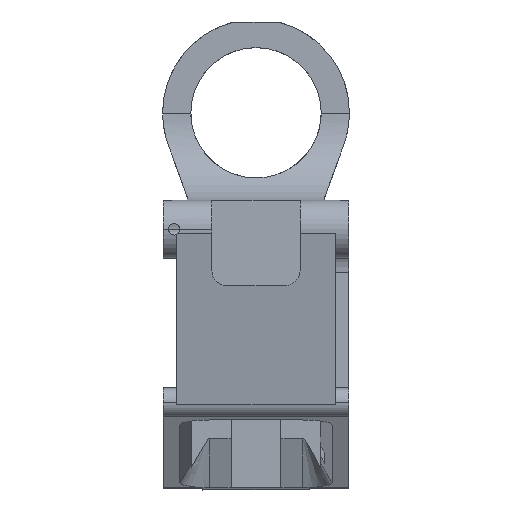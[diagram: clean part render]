
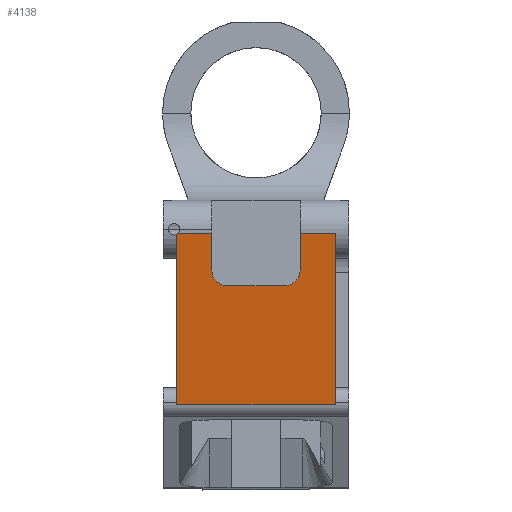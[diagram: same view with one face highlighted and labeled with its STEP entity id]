
A CAD part, top view. The second image highlights one B-rep face of the part: STEP entity #4138.
In plain terms, the highlighted planar face has unit normal (0, -0.156, 0.988).
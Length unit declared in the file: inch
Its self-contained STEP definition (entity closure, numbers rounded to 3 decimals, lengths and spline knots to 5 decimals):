
#20 = CARTESIAN_POINT ( 'NONE',  ( -0.67032, -0.28911, 8.96692 ) ) ;
#81 = EDGE_LOOP ( 'NONE', ( #6582, #3793, #6591, #2601, #5890, #3382, #1505, #7975, #5842, #2264, #7993 ) ) ;
#239 = EDGE_CURVE ( 'NONE', #453, #8430, #6435, .T. ) ;
#329 = DIRECTION ( 'NONE',  ( 0., -0.988, -0.156 ) ) ;
#437 = CARTESIAN_POINT ( 'NONE',  ( 0.675, -1.01855, 8.85139 ) ) ;
#453 = VERTEX_POINT ( 'NONE', #8779 ) ;
#576 = CARTESIAN_POINT ( 'NONE',  ( -0.376, -0.605, 8.91689 ) ) ;
#686 = VERTEX_POINT ( 'NONE', #1953 ) ;
#732 = VERTEX_POINT ( 'NONE', #1987 ) ;
#1032 = EDGE_CURVE ( 'NONE', #8430, #732, #4362, .T. ) ;
#1067 = FACE_OUTER_BOUND ( 'NONE', #81, .T. ) ;
#1092 = CARTESIAN_POINT ( 'NONE',  ( -0.675, -1.74799, 8.73586 ) ) ;
#1142 = CARTESIAN_POINT ( 'NONE',  ( -0.675, -0.29215, 8.96643 ) ) ;
#1505 = ORIENTED_EDGE ( 'NONE', *, *, #6624, .T. ) ;
#1625 = DIRECTION ( 'NONE',  ( 1., 0., 0. ) ) ;
#1953 = CARTESIAN_POINT ( 'NONE',  ( 0.675, -0.28911, 8.96692 ) ) ;
#1987 = CARTESIAN_POINT ( 'NONE',  ( -0.251, -0.73, 8.89709 ) ) ;
#2120 = CARTESIAN_POINT ( 'NONE',  ( 0.376, -0.28911, 8.96692 ) ) ;
#2230 = VERTEX_POINT ( 'NONE', #7194 ) ;
#2264 = ORIENTED_EDGE ( 'NONE', *, *, #239, .T. ) ;
#2399 = VECTOR ( 'NONE', #8054, 39.37008 ) ;
#2515 = CARTESIAN_POINT ( 'NONE',  ( -0.675, -0.28911, 8.96692 ) ) ;
#2586 = CARTESIAN_POINT ( 'NONE',  ( 0.675, -1.74799, 8.73586 ) ) ;
#2601 = ORIENTED_EDGE ( 'NONE', *, *, #8705, .T. ) ;
#2766 = CARTESIAN_POINT ( 'NONE',  ( -0.251, -0.73, 8.89709 ) ) ;
#2842 = LINE ( 'NONE', #3835, #3527 ) ;
#2854 = CARTESIAN_POINT ( 'NONE',  ( -0.675, -1.74799, 8.73586 ) ) ;
#2950 = CARTESIAN_POINT ( 'NONE',  ( -0.675, -0.29215, 8.96643 ) ) ;
#3178 = LINE ( 'NONE', #7490, #8582 ) ;
#3382 = ORIENTED_EDGE ( 'NONE', *, *, #5955, .T. ) ;
#3527 = VECTOR ( 'NONE', #1625, 39.37008 ) ;
#3793 = ORIENTED_EDGE ( 'NONE', *, *, #5943, .T. ) ;
#3835 = CARTESIAN_POINT ( 'NONE',  ( 0., -1.74799, 8.73586 ) ) ;
#3979 = PLANE ( 'NONE',  #4815 ) ;
#4124 = CARTESIAN_POINT ( 'NONE',  ( -0.376, -0.605, 8.91689 ) ) ;
#4138 = ADVANCED_FACE ( 'NONE', ( #1067 ), #3979, .T. ) ;
#4331 = DIRECTION ( 'NONE',  ( 0., 0.988, 0.156 ) ) ;
#4334 = CARTESIAN_POINT ( 'NONE',  ( 0., -0.73, 8.89709 ) ) ;
#4347 = CARTESIAN_POINT ( 'NONE',  ( 0.32422, -0.73, 8.89709 ) ) ;
#4362 = LINE ( 'NONE', #4334, #2399 ) ;
#4546 = CARTESIAN_POINT ( 'NONE',  ( -0.376, -0.28911, 8.96692 ) ) ;
#4596 = VECTOR ( 'NONE', #4825, 39.37008 ) ;
#4651 = VERTEX_POINT ( 'NONE', #1142 ) ;
#4663 = LINE ( 'NONE', #7784, #8807 ) ;
#4726 = DIRECTION ( 'NONE',  ( 0., -0.156, 0.988 ) ) ;
#4778 = VERTEX_POINT ( 'NONE', #2120 ) ;
#4786 =( BOUNDED_CURVE ( )  B_SPLINE_CURVE ( 3, ( #20, #5139, #7344, #2950 ),
 .UNSPECIFIED., .F., .F. ) 
 B_SPLINE_CURVE_WITH_KNOTS ( ( 4, 4 ),
 ( 5.65037, 5.76554 ),
 .UNSPECIFIED. ) 
 CURVE ( )  GEOMETRIC_REPRESENTATION_ITEM ( )  RATIONAL_B_SPLINE_CURVE ( ( 1., 0.999, 0.999, 1. ) ) 
 REPRESENTATION_ITEM ( '' )  );
#4815 = AXIS2_PLACEMENT_3D ( 'NONE', #2515, #4726, #329 ) ;
#4825 = DIRECTION ( 'NONE',  ( 0., 0.988, 0.156 ) ) ;
#4944 = VERTEX_POINT ( 'NONE', #8929 ) ;
#4971 = CARTESIAN_POINT ( 'NONE',  ( -0.376, -0.67822, 8.90529 ) ) ;
#5139 = CARTESIAN_POINT ( 'NONE',  ( -0.67182, -0.29021, 8.96675 ) ) ;
#5152 =( BOUNDED_CURVE ( )  B_SPLINE_CURVE ( 3, ( #2766, #7145, #4971, #576 ),
 .UNSPECIFIED., .F., .F. ) 
 B_SPLINE_CURVE_WITH_KNOTS ( ( 4, 4 ),
 ( 3.14159, 4.71239 ),
 .UNSPECIFIED. ) 
 CURVE ( )  GEOMETRIC_REPRESENTATION_ITEM ( )  RATIONAL_B_SPLINE_CURVE ( ( 1., 0.805, 0.805, 1. ) ) 
 REPRESENTATION_ITEM ( '' )  );
#5331 = CARTESIAN_POINT ( 'NONE',  ( 0.58425, -0.28911, 8.96692 ) ) ;
#5630 = EDGE_CURVE ( 'NONE', #2230, #4944, #3178, .T. ) ;
#5828 = CARTESIAN_POINT ( 'NONE',  ( 0.376, -0.605, 8.91689 ) ) ;
#5842 = ORIENTED_EDGE ( 'NONE', *, *, #7772, .F. ) ;
#5890 = ORIENTED_EDGE ( 'NONE', *, *, #9008, .F. ) ;
#5943 = EDGE_CURVE ( 'NONE', #8506, #2230, #8701, .T. ) ;
#5955 = EDGE_CURVE ( 'NONE', #7697, #8208, #2842, .T. ) ;
#6251 = CARTESIAN_POINT ( 'NONE',  ( 0.251, -0.73, 8.89709 ) ) ;
#6435 =( BOUNDED_CURVE ( )  B_SPLINE_CURVE ( 3, ( #5828, #6515, #4347, #8540 ),
 .UNSPECIFIED., .F., .F. ) 
 B_SPLINE_CURVE_WITH_KNOTS ( ( 4, 4 ),
 ( 4.71239, 6.28319 ),
 .UNSPECIFIED. ) 
 CURVE ( )  GEOMETRIC_REPRESENTATION_ITEM ( )  RATIONAL_B_SPLINE_CURVE ( ( 1., 0.805, 0.805, 1. ) ) 
 REPRESENTATION_ITEM ( '' )  );
#6515 = CARTESIAN_POINT ( 'NONE',  ( 0.376, -0.67822, 8.90529 ) ) ;
#6550 = LINE ( 'NONE', #437, #4596 ) ;
#6582 = ORIENTED_EDGE ( 'NONE', *, *, #8573, .T. ) ;
#6591 = ORIENTED_EDGE ( 'NONE', *, *, #5630, .T. ) ;
#6624 = EDGE_CURVE ( 'NONE', #8208, #686, #6550, .T. ) ;
#6708 = LINE ( 'NONE', #2854, #8426 ) ;
#6736 = VECTOR ( 'NONE', #6752, 39.37008 ) ;
#6752 = DIRECTION ( 'NONE',  ( 0., 0.988, 0.156 ) ) ;
#7145 = CARTESIAN_POINT ( 'NONE',  ( -0.32422, -0.73, 8.89709 ) ) ;
#7194 = CARTESIAN_POINT ( 'NONE',  ( -0.376, -0.28911, 8.96692 ) ) ;
#7344 = CARTESIAN_POINT ( 'NONE',  ( -0.67338, -0.29122, 8.96659 ) ) ;
#7490 = CARTESIAN_POINT ( 'NONE',  ( 0., -0.28911, 8.96692 ) ) ;
#7697 = VERTEX_POINT ( 'NONE', #1092 ) ;
#7772 = EDGE_CURVE ( 'NONE', #453, #4778, #4663, .T. ) ;
#7784 = CARTESIAN_POINT ( 'NONE',  ( 0.376, -0.605, 8.91689 ) ) ;
#7975 = ORIENTED_EDGE ( 'NONE', *, *, #8151, .T. ) ;
#7993 = ORIENTED_EDGE ( 'NONE', *, *, #1032, .T. ) ;
#8054 = DIRECTION ( 'NONE',  ( -1., 0., 0. ) ) ;
#8151 = EDGE_CURVE ( 'NONE', #686, #4778, #9235, .T. ) ;
#8208 = VERTEX_POINT ( 'NONE', #2586 ) ;
#8216 = DIRECTION ( 'NONE',  ( -1., 0., 0. ) ) ;
#8426 = VECTOR ( 'NONE', #4331, 39.37008 ) ;
#8430 = VERTEX_POINT ( 'NONE', #6251 ) ;
#8506 = VERTEX_POINT ( 'NONE', #4124 ) ;
#8527 = DIRECTION ( 'NONE',  ( 0., 0.988, 0.156 ) ) ;
#8540 = CARTESIAN_POINT ( 'NONE',  ( 0.251, -0.73, 8.89709 ) ) ;
#8573 = EDGE_CURVE ( 'NONE', #732, #8506, #5152, .T. ) ;
#8582 = VECTOR ( 'NONE', #8216, 39.37008 ) ;
#8701 = LINE ( 'NONE', #4546, #6736 ) ;
#8705 = EDGE_CURVE ( 'NONE', #4944, #4651, #4786, .T. ) ;
#8779 = CARTESIAN_POINT ( 'NONE',  ( 0.376, -0.605, 8.91689 ) ) ;
#8807 = VECTOR ( 'NONE', #8527, 39.37008 ) ;
#8929 = CARTESIAN_POINT ( 'NONE',  ( -0.67032, -0.28911, 8.96692 ) ) ;
#8977 = DIRECTION ( 'NONE',  ( -1., 0., 0. ) ) ;
#9008 = EDGE_CURVE ( 'NONE', #7697, #4651, #6708, .T. ) ;
#9016 = VECTOR ( 'NONE', #8977, 39.37008 ) ;
#9235 = LINE ( 'NONE', #5331, #9016 ) ;
